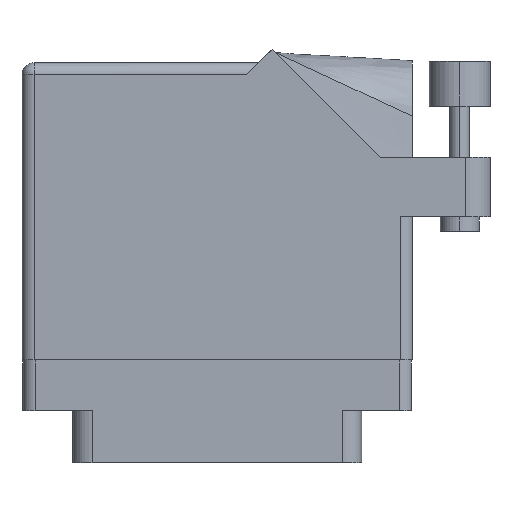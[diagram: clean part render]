
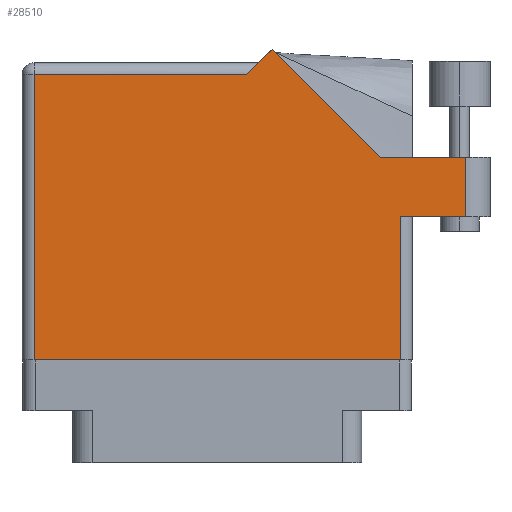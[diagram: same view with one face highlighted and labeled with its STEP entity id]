
A CAD part, front view. The second image highlights one B-rep face of the part: STEP entity #28510.
In plain terms, the highlighted face is planar.
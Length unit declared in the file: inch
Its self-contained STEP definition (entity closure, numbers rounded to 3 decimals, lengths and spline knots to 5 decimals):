
#598 = DIRECTION ( 'NONE',  ( -1., 0., 0. ) ) ;
#916 = CARTESIAN_POINT ( 'NONE',  ( 1.217, 1.53, 0. ) ) ;
#1257 = DIRECTION ( 'NONE',  ( -1., 0., 0. ) ) ;
#1301 = LINE ( 'NONE', #37972, #28560 ) ;
#1371 = VECTOR ( 'NONE', #37910, 39.37008 ) ;
#1891 = VECTOR ( 'NONE', #12818, 39.37008 ) ;
#1941 = CARTESIAN_POINT ( 'NONE',  ( 0., 0., 0. ) ) ;
#2192 = VERTEX_POINT ( 'NONE', #11878 ) ;
#2331 = LINE ( 'NONE', #19119, #1891 ) ;
#5631 = VECTOR ( 'NONE', #1257, 39.37008 ) ;
#5812 = AXIS2_PLACEMENT_3D ( 'NONE', #16051, #37035, #598 ) ;
#6567 = FACE_OUTER_BOUND ( 'NONE', #8789, .T. ) ;
#6685 = EDGE_CURVE ( 'NONE', #27127, #31494, #19404, .T. ) ;
#6729 = CARTESIAN_POINT ( 'NONE',  ( 2.285, 1.044, 0. ) ) ;
#6793 = ORIENTED_EDGE ( 'NONE', *, *, #34571, .T. ) ;
#7394 = EDGE_CURVE ( 'NONE', #35362, #2192, #36215, .T. ) ;
#8105 = CARTESIAN_POINT ( 'NONE',  ( 2.285, 1.044, 0. ) ) ;
#8687 = CARTESIAN_POINT ( 'NONE',  ( 1.84442, 1.044, 0. ) ) ;
#8789 = EDGE_LOOP ( 'NONE', ( #30855, #29575, #35050, #20192, #6793, #10481, #10344, #21284, #37873 ) ) ;
#9247 = DIRECTION ( 'NONE',  ( -1., 0., 0. ) ) ;
#10344 = ORIENTED_EDGE ( 'NONE', *, *, #38046, .T. ) ;
#10481 = ORIENTED_EDGE ( 'NONE', *, *, #6685, .T. ) ;
#11243 = DIRECTION ( 'NONE',  ( 1., 0., 0. ) ) ;
#11878 = CARTESIAN_POINT ( 'NONE',  ( 1.28771, 1.60071, 0. ) ) ;
#12495 = LINE ( 'NONE', #29256, #32235 ) ;
#12503 = CARTESIAN_POINT ( 'NONE',  ( 0.062, 0., 0. ) ) ;
#12818 = DIRECTION ( 'NONE',  ( 0., -1., 0. ) ) ;
#13662 = CARTESIAN_POINT ( 'NONE',  ( 2.41, 1.044, 0. ) ) ;
#15146 = VERTEX_POINT ( 'NONE', #6729 ) ;
#15501 = VERTEX_POINT ( 'NONE', #33315 ) ;
#16051 = CARTESIAN_POINT ( 'NONE',  ( 0., 1.53, 0. ) ) ;
#17125 = EDGE_CURVE ( 'NONE', #33190, #28034, #12495, .T. ) ;
#17337 = VECTOR ( 'NONE', #20245, 39.37008 ) ;
#17400 = CARTESIAN_POINT ( 'NONE',  ( 1.155, 1.468, 0. ) ) ;
#19079 = VECTOR ( 'NONE', #33693, 39.37008 ) ;
#19119 = CARTESIAN_POINT ( 'NONE',  ( 0.062, 0., 0. ) ) ;
#19186 = PLANE ( 'NONE',  #5812 ) ;
#19404 = LINE ( 'NONE', #36002, #37716 ) ;
#20192 = ORIENTED_EDGE ( 'NONE', *, *, #7394, .T. ) ;
#20245 = DIRECTION ( 'NONE',  ( 1., 0., 0. ) ) ;
#21271 = EDGE_CURVE ( 'NONE', #38512, #15501, #25399, .T. ) ;
#21284 = ORIENTED_EDGE ( 'NONE', *, *, #21271, .T. ) ;
#25399 = LINE ( 'NONE', #1941, #17337 ) ;
#26916 = EDGE_CURVE ( 'NONE', #28034, #15146, #36603, .T. ) ;
#27127 = VERTEX_POINT ( 'NONE', #17400 ) ;
#27373 = DIRECTION ( 'NONE',  ( -0.707, 0.707, 0. ) ) ;
#28034 = VERTEX_POINT ( 'NONE', #37216 ) ;
#28434 = CARTESIAN_POINT ( 'NONE',  ( 1.948, 0.737, 0. ) ) ;
#28510 = ADVANCED_FACE ( 'NONE', ( #6567 ), #19186, .F. ) ;
#28560 = VECTOR ( 'NONE', #29201, 39.37008 ) ;
#28598 = EDGE_CURVE ( 'NONE', #15146, #35362, #32471, .T. ) ;
#29201 = DIRECTION ( 'NONE',  ( 0., 1., 0. ) ) ;
#29256 = CARTESIAN_POINT ( 'NONE',  ( 2.01, 0.737, 0. ) ) ;
#29575 = ORIENTED_EDGE ( 'NONE', *, *, #26916, .T. ) ;
#30855 = ORIENTED_EDGE ( 'NONE', *, *, #17125, .T. ) ;
#31298 = CARTESIAN_POINT ( 'NONE',  ( 1.84442, 1.044, 0. ) ) ;
#31494 = VERTEX_POINT ( 'NONE', #38474 ) ;
#32235 = VECTOR ( 'NONE', #11243, 39.37008 ) ;
#32471 = LINE ( 'NONE', #13662, #5631 ) ;
#33190 = VERTEX_POINT ( 'NONE', #28434 ) ;
#33315 = CARTESIAN_POINT ( 'NONE',  ( 1.948, 0., 0. ) ) ;
#33693 = DIRECTION ( 'NONE',  ( -0.707, -0.707, 0. ) ) ;
#34301 = EDGE_CURVE ( 'NONE', #15501, #33190, #1301, .T. ) ;
#34343 = VECTOR ( 'NONE', #27373, 39.37008 ) ;
#34571 = EDGE_CURVE ( 'NONE', #2192, #27127, #36433, .T. ) ;
#35050 = ORIENTED_EDGE ( 'NONE', *, *, #28598, .T. ) ;
#35362 = VERTEX_POINT ( 'NONE', #31298 ) ;
#36002 = CARTESIAN_POINT ( 'NONE',  ( 0., 1.468, 0. ) ) ;
#36215 = LINE ( 'NONE', #8687, #34343 ) ;
#36433 = LINE ( 'NONE', #916, #19079 ) ;
#36603 = LINE ( 'NONE', #8105, #1371 ) ;
#37035 = DIRECTION ( 'NONE',  ( 0., 0., -1. ) ) ;
#37216 = CARTESIAN_POINT ( 'NONE',  ( 2.285, 0.737, 0. ) ) ;
#37716 = VECTOR ( 'NONE', #9247, 39.37008 ) ;
#37873 = ORIENTED_EDGE ( 'NONE', *, *, #34301, .T. ) ;
#37910 = DIRECTION ( 'NONE',  ( 0., 1., 0. ) ) ;
#37972 = CARTESIAN_POINT ( 'NONE',  ( 1.948, 0.737, 0. ) ) ;
#38046 = EDGE_CURVE ( 'NONE', #31494, #38512, #2331, .T. ) ;
#38474 = CARTESIAN_POINT ( 'NONE',  ( 0.062, 1.468, 0. ) ) ;
#38512 = VERTEX_POINT ( 'NONE', #12503 ) ;
